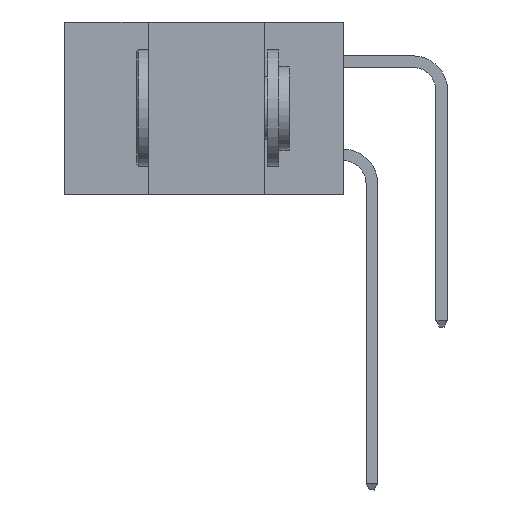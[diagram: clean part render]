
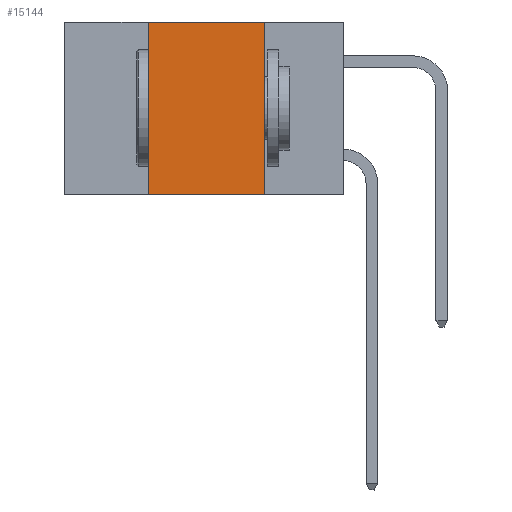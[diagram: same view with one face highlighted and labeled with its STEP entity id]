
A CAD part, left-side view. The second image highlights one B-rep face of the part: STEP entity #15144.
In plain terms, the highlighted planar face has unit normal (-1, 0, 0).
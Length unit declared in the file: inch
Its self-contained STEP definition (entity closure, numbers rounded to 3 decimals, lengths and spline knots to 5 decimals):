
#618 = AXIS2_PLACEMENT_3D ( 'NONE', #11675, #11642, #11610 ) ;
#2722 = EDGE_LOOP ( 'NONE', ( #3466, #4160, #5612, #6172 ) ) ;
#3466 = ORIENTED_EDGE ( 'NONE', *, *, #15186, .F. ) ;
#3719 = CARTESIAN_POINT ( 'NONE',  ( 0., 0.42, 0. ) ) ;
#4160 = ORIENTED_EDGE ( 'NONE', *, *, #14296, .F. ) ;
#4176 = CARTESIAN_POINT ( 'NONE',  ( 0., 0.6, 0. ) ) ;
#4980 = VERTEX_POINT ( 'NONE', #3719 ) ;
#5307 = CARTESIAN_POINT ( 'NONE',  ( 0., 0.6, -0.37 ) ) ;
#5612 = ORIENTED_EDGE ( 'NONE', *, *, #11643, .F. ) ;
#6031 = LINE ( 'NONE', #5307, #12390 ) ;
#6107 = DIRECTION ( 'NONE',  ( 0., -1., 0. ) ) ;
#6172 = ORIENTED_EDGE ( 'NONE', *, *, #10747, .T. ) ;
#6388 = VERTEX_POINT ( 'NONE', #14192 ) ;
#7052 = CARTESIAN_POINT ( 'NONE',  ( 0., 0.17, 0. ) ) ;
#7188 = LINE ( 'NONE', #11289, #13512 ) ;
#7506 = VECTOR ( 'NONE', #13498, 39.37008 ) ;
#9587 = LINE ( 'NONE', #4176, #12708 ) ;
#10392 = FACE_OUTER_BOUND ( 'NONE', #2722, .T. ) ;
#10747 = EDGE_CURVE ( 'NONE', #6388, #14993, #6031, .T. ) ;
#11289 = CARTESIAN_POINT ( 'NONE',  ( 0., 0.17, -0.37 ) ) ;
#11312 = DIRECTION ( 'NONE',  ( 0., 0., -1. ) ) ;
#11610 = DIRECTION ( 'NONE',  ( 0., 0., -1. ) ) ;
#11642 = DIRECTION ( 'NONE',  ( 1., 0., 0. ) ) ;
#11643 = EDGE_CURVE ( 'NONE', #6388, #4980, #14625, .T. ) ;
#11675 = CARTESIAN_POINT ( 'NONE',  ( 0., 0.6, 0. ) ) ;
#11905 = PLANE ( 'NONE',  #618 ) ;
#12390 = VECTOR ( 'NONE', #6107, 39.37008 ) ;
#12708 = VECTOR ( 'NONE', #16148, 39.37008 ) ;
#13498 = DIRECTION ( 'NONE',  ( 0., 0., 1. ) ) ;
#13512 = VECTOR ( 'NONE', #11312, 39.37008 ) ;
#14192 = CARTESIAN_POINT ( 'NONE',  ( 0., 0.42, -0.37 ) ) ;
#14296 = EDGE_CURVE ( 'NONE', #4980, #15620, #9587, .T. ) ;
#14625 = LINE ( 'NONE', #15810, #7506 ) ;
#14993 = VERTEX_POINT ( 'NONE', #15836 ) ;
#15144 = ADVANCED_FACE ( 'NONE', ( #10392 ), #11905, .F. ) ;
#15186 = EDGE_CURVE ( 'NONE', #15620, #14993, #7188, .T. ) ;
#15620 = VERTEX_POINT ( 'NONE', #7052 ) ;
#15810 = CARTESIAN_POINT ( 'NONE',  ( 0., 0.42, -0.37 ) ) ;
#15836 = CARTESIAN_POINT ( 'NONE',  ( 0., 0.17, -0.37 ) ) ;
#16148 = DIRECTION ( 'NONE',  ( 0., -1., 0. ) ) ;
